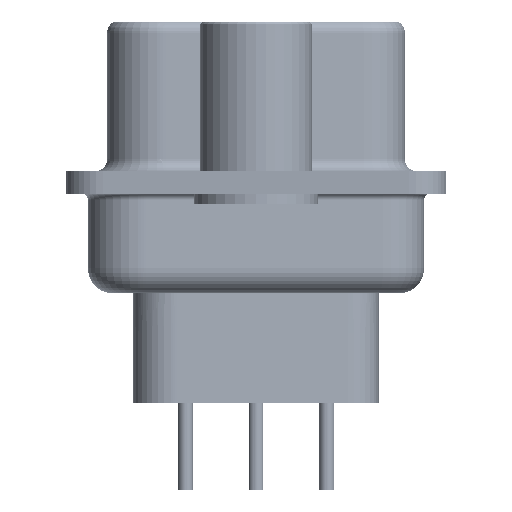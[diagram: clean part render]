
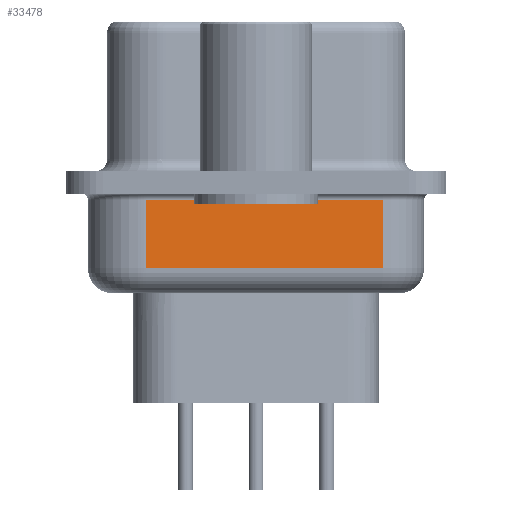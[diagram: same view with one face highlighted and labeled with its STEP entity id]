
A CAD part, left-side view. The second image highlights one B-rep face of the part: STEP entity #33478.
In plain terms, the highlighted planar face has unit normal (-0.985, -0.174, 0).
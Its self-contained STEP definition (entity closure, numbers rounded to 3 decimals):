
#2622 = DIRECTION ( 'NONE',  ( -0.174, 0.985, 0. ) ) ;
#3331 = DIRECTION ( 'NONE',  ( 0., 0., 1. ) ) ;
#4121 = DIRECTION ( 'NONE',  ( 0., 0., 1. ) ) ;
#8046 = CARTESIAN_POINT ( 'NONE',  ( 2.93, 4.403, -4.45 ) ) ;
#8340 = VERTEX_POINT ( 'NONE', #9667 ) ;
#8819 = PLANE ( 'NONE',  #37013 ) ;
#9024 = FACE_OUTER_BOUND ( 'NONE', #37952, .T. ) ;
#9078 = CARTESIAN_POINT ( 'NONE',  ( 2.93, 4.403, -3.45 ) ) ;
#9286 = ORIENTED_EDGE ( 'NONE', *, *, #18335, .F. ) ;
#9667 = CARTESIAN_POINT ( 'NONE',  ( 2.93, 4.403, -0.7 ) ) ;
#10713 = CARTESIAN_POINT ( 'NONE',  ( 4.605, -5.097, -0.7 ) ) ;
#12483 = VECTOR ( 'NONE', #21687, 1000. ) ;
#13435 = EDGE_CURVE ( 'NONE', #32403, #24494, #28092, .T. ) ;
#14952 = VERTEX_POINT ( 'NONE', #10713 ) ;
#15020 = DIRECTION ( 'NONE',  ( 0.985, 0.174, 0. ) ) ;
#18026 = VECTOR ( 'NONE', #4121, 1000. ) ;
#18335 = EDGE_CURVE ( 'NONE', #32403, #8340, #19818, .T. ) ;
#19818 = LINE ( 'NONE', #8046, #18026 ) ;
#20917 = CARTESIAN_POINT ( 'NONE',  ( 2.93, 4.403, -3.45 ) ) ;
#21687 = DIRECTION ( 'NONE',  ( 0.174, -0.985, 0. ) ) ;
#23333 = CARTESIAN_POINT ( 'NONE',  ( 4.605, -5.097, -3.45 ) ) ;
#23355 = CARTESIAN_POINT ( 'NONE',  ( 2.93, 4.403, -0.7 ) ) ;
#23723 = ORIENTED_EDGE ( 'NONE', *, *, #13435, .T. ) ;
#24331 = ORIENTED_EDGE ( 'NONE', *, *, #33973, .T. ) ;
#24494 = VERTEX_POINT ( 'NONE', #23333 ) ;
#28092 = LINE ( 'NONE', #9078, #12483 ) ;
#28144 = CARTESIAN_POINT ( 'NONE',  ( 4.605, -5.097, -4.45 ) ) ;
#30726 = CARTESIAN_POINT ( 'NONE',  ( 2.93, 4.403, -4.45 ) ) ;
#31242 = LINE ( 'NONE', #28144, #37054 ) ;
#32403 = VERTEX_POINT ( 'NONE', #20917 ) ;
#32739 = EDGE_CURVE ( 'NONE', #14952, #8340, #39029, .T. ) ;
#33478 = ADVANCED_FACE ( 'NONE', ( #9024 ), #8819, .F. ) ;
#33973 = EDGE_CURVE ( 'NONE', #24494, #14952, #31242, .T. ) ;
#35942 = DIRECTION ( 'NONE',  ( -0.174, 0.985, 0. ) ) ;
#36498 = ORIENTED_EDGE ( 'NONE', *, *, #32739, .T. ) ;
#37013 = AXIS2_PLACEMENT_3D ( 'NONE', #30726, #15020, #2622 ) ;
#37054 = VECTOR ( 'NONE', #3331, 1000. ) ;
#37952 = EDGE_LOOP ( 'NONE', ( #9286, #23723, #24331, #36498 ) ) ;
#38354 = VECTOR ( 'NONE', #35942, 1000. ) ;
#39029 = LINE ( 'NONE', #23355, #38354 ) ;
